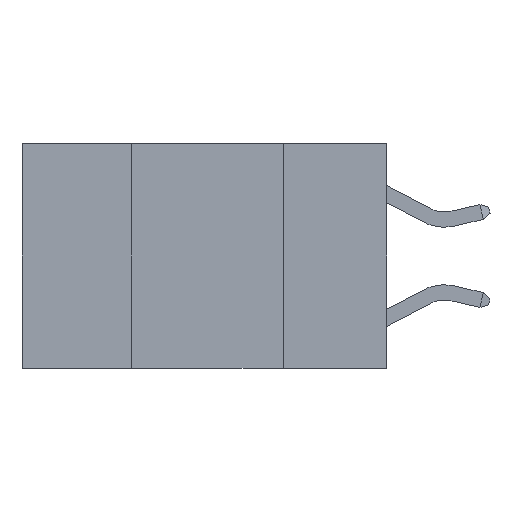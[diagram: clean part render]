
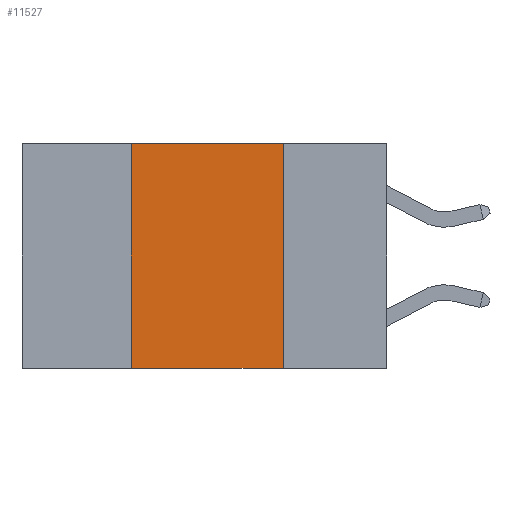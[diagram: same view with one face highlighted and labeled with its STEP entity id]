
A CAD part, left-side view. The second image highlights one B-rep face of the part: STEP entity #11527.
In plain terms, the highlighted planar face has unit normal (-1, 0, 0).
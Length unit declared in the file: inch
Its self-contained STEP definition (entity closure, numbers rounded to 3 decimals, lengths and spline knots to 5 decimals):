
#1132 = EDGE_CURVE ( 'NONE', #6644, #27982, #11413, .T. ) ;
#1891 = VERTEX_POINT ( 'NONE', #15355 ) ;
#1892 = PLANE ( 'NONE',  #25400 ) ;
#2001 = ORIENTED_EDGE ( 'NONE', *, *, #27005, .F. ) ;
#2519 = CARTESIAN_POINT ( 'NONE',  ( 0., 0.17, 0. ) ) ;
#3174 = CARTESIAN_POINT ( 'NONE',  ( 0., 0.42, 0. ) ) ;
#3997 = EDGE_LOOP ( 'NONE', ( #24532, #2001, #14404, #26693 ) ) ;
#4262 = DIRECTION ( 'NONE',  ( 0., 0., -1. ) ) ;
#4898 = DIRECTION ( 'NONE',  ( 0., 0., -1. ) ) ;
#4946 = CARTESIAN_POINT ( 'NONE',  ( 0., 0.6, 0. ) ) ;
#5534 = DIRECTION ( 'NONE',  ( 0., 0., 1. ) ) ;
#5984 = DIRECTION ( 'NONE',  ( 0., -1., 0. ) ) ;
#6129 = VECTOR ( 'NONE', #23530, 39.37008 ) ;
#6644 = VERTEX_POINT ( 'NONE', #22981 ) ;
#10671 = FACE_OUTER_BOUND ( 'NONE', #3997, .T. ) ;
#11015 = VECTOR ( 'NONE', #4898, 39.37008 ) ;
#11413 = LINE ( 'NONE', #3174, #16146 ) ;
#11527 = ADVANCED_FACE ( 'NONE', ( #10671 ), #1892, .F. ) ;
#12305 = LINE ( 'NONE', #4946, #6129 ) ;
#14404 = ORIENTED_EDGE ( 'NONE', *, *, #1132, .F. ) ;
#15355 = CARTESIAN_POINT ( 'NONE',  ( 0., 0.17, -0.37 ) ) ;
#16146 = VECTOR ( 'NONE', #5534, 39.37008 ) ;
#17137 = CARTESIAN_POINT ( 'NONE',  ( 0., 0.17, 0. ) ) ;
#18192 = DIRECTION ( 'NONE',  ( 1., 0., 0. ) ) ;
#18721 = VECTOR ( 'NONE', #5984, 39.37008 ) ;
#19293 = EDGE_CURVE ( 'NONE', #27155, #1891, #29430, .T. ) ;
#22232 = CARTESIAN_POINT ( 'NONE',  ( 0., 0.6, -0.37 ) ) ;
#22306 = EDGE_CURVE ( 'NONE', #6644, #1891, #29508, .T. ) ;
#22981 = CARTESIAN_POINT ( 'NONE',  ( 0., 0.42, -0.37 ) ) ;
#23530 = DIRECTION ( 'NONE',  ( 0., -1., 0. ) ) ;
#24532 = ORIENTED_EDGE ( 'NONE', *, *, #19293, .F. ) ;
#25035 = CARTESIAN_POINT ( 'NONE',  ( 0., 0.6, 0. ) ) ;
#25400 = AXIS2_PLACEMENT_3D ( 'NONE', #25035, #18192, #4262 ) ;
#26693 = ORIENTED_EDGE ( 'NONE', *, *, #22306, .T. ) ;
#27005 = EDGE_CURVE ( 'NONE', #27982, #27155, #12305, .T. ) ;
#27155 = VERTEX_POINT ( 'NONE', #17137 ) ;
#27982 = VERTEX_POINT ( 'NONE', #29077 ) ;
#29077 = CARTESIAN_POINT ( 'NONE',  ( 0., 0.42, 0. ) ) ;
#29430 = LINE ( 'NONE', #2519, #11015 ) ;
#29508 = LINE ( 'NONE', #22232, #18721 ) ;
